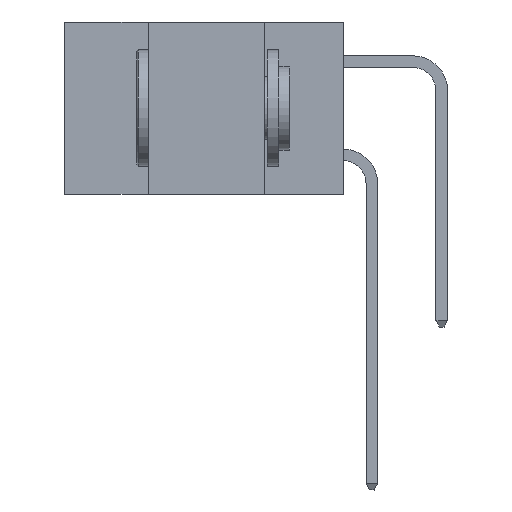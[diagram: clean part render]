
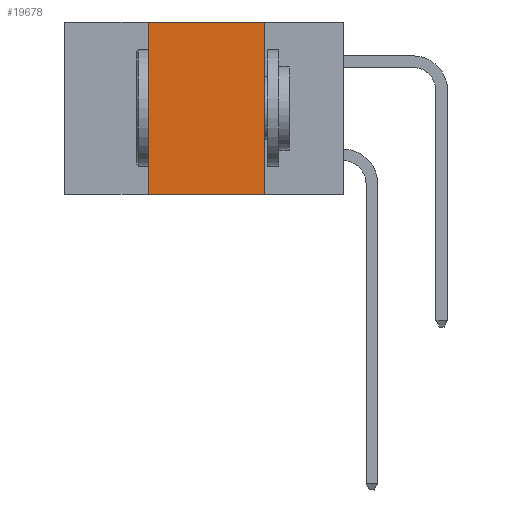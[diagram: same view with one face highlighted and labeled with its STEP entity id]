
A CAD part, left-side view. The second image highlights one B-rep face of the part: STEP entity #19678.
In plain terms, the highlighted planar face has unit normal (-1, 0, 0).
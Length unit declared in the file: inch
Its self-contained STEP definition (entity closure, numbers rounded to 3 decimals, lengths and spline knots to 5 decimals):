
#2304 = VECTOR ( 'NONE', #18198, 39.37008 ) ;
#3534 = CARTESIAN_POINT ( 'NONE',  ( 0., 0.17, 0. ) ) ;
#3787 = ORIENTED_EDGE ( 'NONE', *, *, #12111, .F. ) ;
#4282 = PLANE ( 'NONE',  #26711 ) ;
#4635 = FACE_OUTER_BOUND ( 'NONE', #15685, .T. ) ;
#4867 = CARTESIAN_POINT ( 'NONE',  ( 0., 0.42, -0.37 ) ) ;
#5158 = CARTESIAN_POINT ( 'NONE',  ( 0., 0.42, 0. ) ) ;
#7432 = LINE ( 'NONE', #3534, #11713 ) ;
#8060 = CARTESIAN_POINT ( 'NONE',  ( 0., 0.17, 0. ) ) ;
#9298 = DIRECTION ( 'NONE',  ( 0., 0., -1. ) ) ;
#9567 = VECTOR ( 'NONE', #22733, 39.37008 ) ;
#9763 = LINE ( 'NONE', #10578, #2304 ) ;
#10578 = CARTESIAN_POINT ( 'NONE',  ( 0., 0.6, -0.37 ) ) ;
#11713 = VECTOR ( 'NONE', #18686, 39.37008 ) ;
#12111 = EDGE_CURVE ( 'NONE', #17877, #24007, #7432, .T. ) ;
#13767 = VERTEX_POINT ( 'NONE', #4867 ) ;
#15685 = EDGE_LOOP ( 'NONE', ( #3787, #17162, #17573, #29780 ) ) ;
#16289 = LINE ( 'NONE', #5158, #9567 ) ;
#17162 = ORIENTED_EDGE ( 'NONE', *, *, #31910, .F. ) ;
#17278 = CARTESIAN_POINT ( 'NONE',  ( 0., 0.17, -0.37 ) ) ;
#17573 = ORIENTED_EDGE ( 'NONE', *, *, #25642, .F. ) ;
#17877 = VERTEX_POINT ( 'NONE', #8060 ) ;
#18198 = DIRECTION ( 'NONE',  ( 0., -1., 0. ) ) ;
#18686 = DIRECTION ( 'NONE',  ( 0., 0., -1. ) ) ;
#19678 = ADVANCED_FACE ( 'NONE', ( #4635 ), #4282, .F. ) ;
#20810 = LINE ( 'NONE', #30910, #21580 ) ;
#21580 = VECTOR ( 'NONE', #23354, 39.37008 ) ;
#21837 = CARTESIAN_POINT ( 'NONE',  ( 0., 0.6, 0. ) ) ;
#22733 = DIRECTION ( 'NONE',  ( 0., 0., 1. ) ) ;
#23354 = DIRECTION ( 'NONE',  ( 0., -1., 0. ) ) ;
#24007 = VERTEX_POINT ( 'NONE', #17278 ) ;
#24383 = DIRECTION ( 'NONE',  ( 1., 0., 0. ) ) ;
#24888 = VERTEX_POINT ( 'NONE', #26614 ) ;
#25642 = EDGE_CURVE ( 'NONE', #13767, #24888, #16289, .T. ) ;
#26614 = CARTESIAN_POINT ( 'NONE',  ( 0., 0.42, 0. ) ) ;
#26711 = AXIS2_PLACEMENT_3D ( 'NONE', #21837, #24383, #9298 ) ;
#29780 = ORIENTED_EDGE ( 'NONE', *, *, #31835, .T. ) ;
#30910 = CARTESIAN_POINT ( 'NONE',  ( 0., 0.6, 0. ) ) ;
#31835 = EDGE_CURVE ( 'NONE', #13767, #24007, #9763, .T. ) ;
#31910 = EDGE_CURVE ( 'NONE', #24888, #17877, #20810, .T. ) ;
